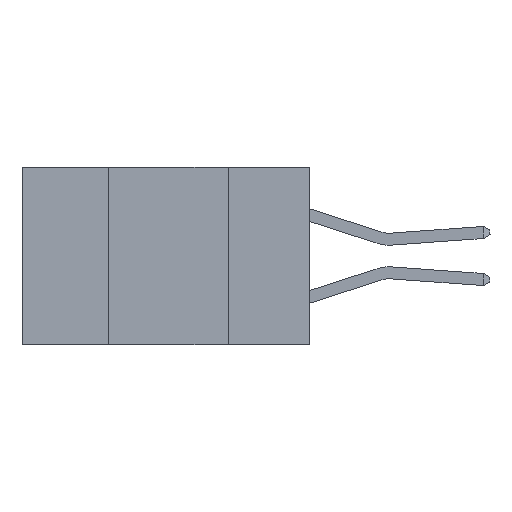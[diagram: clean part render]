
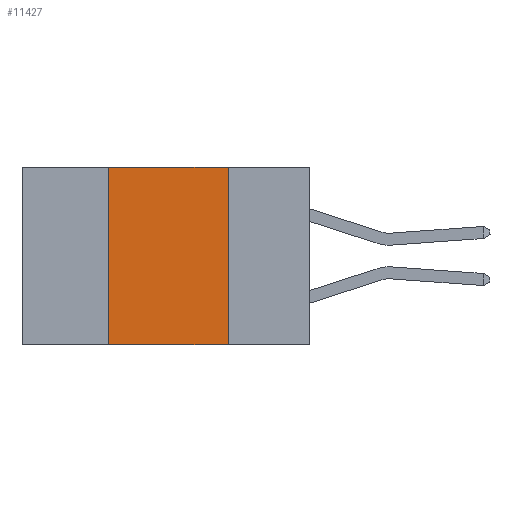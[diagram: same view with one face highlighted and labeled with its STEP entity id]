
A CAD part, left-side view. The second image highlights one B-rep face of the part: STEP entity #11427.
In plain terms, the highlighted planar face has unit normal (-1, 0, 0).
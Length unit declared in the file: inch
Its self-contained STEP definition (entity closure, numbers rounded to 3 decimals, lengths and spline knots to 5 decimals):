
#2403 = LINE ( 'NONE', #16068, #14460 ) ;
#2906 = ORIENTED_EDGE ( 'NONE', *, *, #16069, .T. ) ;
#3530 = LINE ( 'NONE', #29549, #18582 ) ;
#3841 = ORIENTED_EDGE ( 'NONE', *, *, #24273, .F. ) ;
#6224 = DIRECTION ( 'NONE',  ( 1., 0., 0. ) ) ;
#10035 = VERTEX_POINT ( 'NONE', #29227 ) ;
#10267 = ORIENTED_EDGE ( 'NONE', *, *, #14631, .F. ) ;
#10819 = EDGE_CURVE ( 'NONE', #10035, #11125, #2403, .T. ) ;
#10946 = VECTOR ( 'NONE', #20910, 39.37008 ) ;
#11125 = VERTEX_POINT ( 'NONE', #17162 ) ;
#11427 = ADVANCED_FACE ( 'NONE', ( #15541 ), #13415, .F. ) ;
#12607 = AXIS2_PLACEMENT_3D ( 'NONE', #20608, #6224, #22986 ) ;
#12974 = DIRECTION ( 'NONE',  ( 0., -1., 0. ) ) ;
#13415 = PLANE ( 'NONE',  #12607 ) ;
#14460 = VECTOR ( 'NONE', #18427, 39.37008 ) ;
#14631 = EDGE_CURVE ( 'NONE', #25799, #27887, #25006, .T. ) ;
#15541 = FACE_OUTER_BOUND ( 'NONE', #24713, .T. ) ;
#16068 = CARTESIAN_POINT ( 'NONE',  ( 0., 0.17, 0. ) ) ;
#16069 = EDGE_CURVE ( 'NONE', #25799, #11125, #3530, .T. ) ;
#17162 = CARTESIAN_POINT ( 'NONE',  ( 0., 0.17, -0.37 ) ) ;
#18001 = DIRECTION ( 'NONE',  ( 0., 0., 1. ) ) ;
#18427 = DIRECTION ( 'NONE',  ( 0., 0., -1. ) ) ;
#18476 = CARTESIAN_POINT ( 'NONE',  ( 0., 0.6, 0. ) ) ;
#18582 = VECTOR ( 'NONE', #12974, 39.37008 ) ;
#18675 = VECTOR ( 'NONE', #18001, 39.37008 ) ;
#20327 = ORIENTED_EDGE ( 'NONE', *, *, #10819, .F. ) ;
#20608 = CARTESIAN_POINT ( 'NONE',  ( 0., 0.6, 0. ) ) ;
#20910 = DIRECTION ( 'NONE',  ( 0., -1., 0. ) ) ;
#21528 = CARTESIAN_POINT ( 'NONE',  ( 0., 0.42, -0.37 ) ) ;
#22986 = DIRECTION ( 'NONE',  ( 0., 0., -1. ) ) ;
#23204 = CARTESIAN_POINT ( 'NONE',  ( 0., 0.42, 0. ) ) ;
#24273 = EDGE_CURVE ( 'NONE', #27887, #10035, #29882, .T. ) ;
#24713 = EDGE_LOOP ( 'NONE', ( #20327, #3841, #10267, #2906 ) ) ;
#25006 = LINE ( 'NONE', #29811, #18675 ) ;
#25799 = VERTEX_POINT ( 'NONE', #21528 ) ;
#27887 = VERTEX_POINT ( 'NONE', #23204 ) ;
#29227 = CARTESIAN_POINT ( 'NONE',  ( 0., 0.17, 0. ) ) ;
#29549 = CARTESIAN_POINT ( 'NONE',  ( 0., 0.6, -0.37 ) ) ;
#29811 = CARTESIAN_POINT ( 'NONE',  ( 0., 0.42, 0. ) ) ;
#29882 = LINE ( 'NONE', #18476, #10946 ) ;
